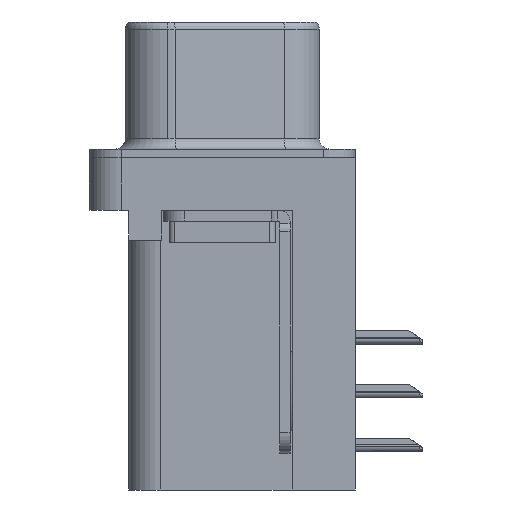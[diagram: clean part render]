
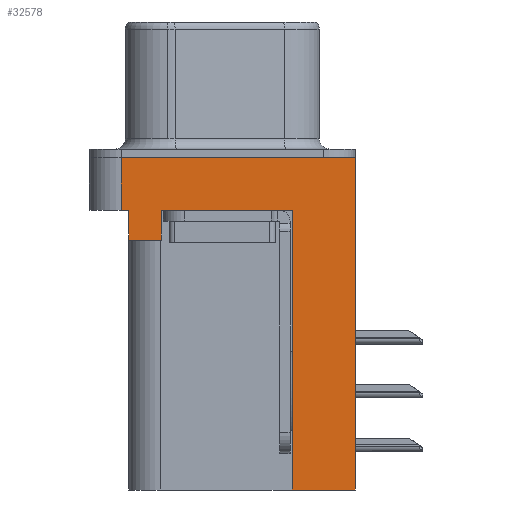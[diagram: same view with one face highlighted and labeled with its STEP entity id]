
A CAD part, left-side view. The second image highlights one B-rep face of the part: STEP entity #32578.
In plain terms, the highlighted planar face has unit normal (-1, 0, 0).
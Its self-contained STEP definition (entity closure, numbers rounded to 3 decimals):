
#447 = VERTEX_POINT ( 'NONE', #12961 ) ;
#768 = EDGE_CURVE ( 'NONE', #20074, #5395, #31731, .T. ) ;
#1675 = LINE ( 'NONE', #16676, #16002 ) ;
#2253 = ORIENTED_EDGE ( 'NONE', *, *, #27687, .T. ) ;
#2618 = ORIENTED_EDGE ( 'NONE', *, *, #26291, .F. ) ;
#2777 = DIRECTION ( 'NONE',  ( 0., 0., 1. ) ) ;
#2835 = CARTESIAN_POINT ( 'NONE',  ( -2.91, -6.275, -2.5 ) ) ;
#2850 = AXIS2_PLACEMENT_3D ( 'NONE', #2835, #25603, #8645 ) ;
#3186 = VECTOR ( 'NONE', #23266, 1000. ) ;
#3810 = LINE ( 'NONE', #24291, #19846 ) ;
#3878 = EDGE_CURVE ( 'NONE', #5395, #35663, #27976, .T. ) ;
#3960 = CARTESIAN_POINT ( 'NONE',  ( -2.91, -6.275, -2.5 ) ) ;
#4113 = LINE ( 'NONE', #3960, #33430 ) ;
#4437 = CARTESIAN_POINT ( 'NONE',  ( -2.91, -6.275, 0. ) ) ;
#5290 = DIRECTION ( 'NONE',  ( 0., 1., 0. ) ) ;
#5320 = EDGE_CURVE ( 'NONE', #447, #14655, #1675, .T. ) ;
#5395 = VERTEX_POINT ( 'NONE', #36560 ) ;
#5920 = VECTOR ( 'NONE', #34049, 1000. ) ;
#6061 = ORIENTED_EDGE ( 'NONE', *, *, #768, .F. ) ;
#6832 = LINE ( 'NONE', #25537, #5920 ) ;
#7365 = DIRECTION ( 'NONE',  ( 0., -1., 0. ) ) ;
#7595 = EDGE_CURVE ( 'NONE', #32643, #447, #21577, .T. ) ;
#7699 = LINE ( 'NONE', #20429, #3186 ) ;
#8645 = DIRECTION ( 'NONE',  ( 0., 0., 1. ) ) ;
#9405 = CARTESIAN_POINT ( 'NONE',  ( -2.91, 2.895, -3.9 ) ) ;
#10199 = DIRECTION ( 'NONE',  ( 0., -1., 0. ) ) ;
#10354 = CARTESIAN_POINT ( 'NONE',  ( -2.91, 4.425, -2.5 ) ) ;
#11674 = FACE_OUTER_BOUND ( 'NONE', #19146, .T. ) ;
#12716 = CARTESIAN_POINT ( 'NONE',  ( -2.91, -6.275, 0. ) ) ;
#12940 = VECTOR ( 'NONE', #7365, 1000. ) ;
#12961 = CARTESIAN_POINT ( 'NONE',  ( -2.91, -3.295, -15.7 ) ) ;
#13712 = DIRECTION ( 'NONE',  ( 0., 0., 1. ) ) ;
#13797 = VERTEX_POINT ( 'NONE', #10354 ) ;
#14472 = VERTEX_POINT ( 'NONE', #16010 ) ;
#14655 = VERTEX_POINT ( 'NONE', #36496 ) ;
#14767 = ORIENTED_EDGE ( 'NONE', *, *, #32955, .F. ) ;
#15121 = CARTESIAN_POINT ( 'NONE',  ( -2.91, 4.425, -3.9 ) ) ;
#16002 = VECTOR ( 'NONE', #13712, 1000. ) ;
#16010 = CARTESIAN_POINT ( 'NONE',  ( -2.91, 4.425, -3.9 ) ) ;
#16676 = CARTESIAN_POINT ( 'NONE',  ( -2.91, -3.295, -15.7 ) ) ;
#17444 = CARTESIAN_POINT ( 'NONE',  ( -2.91, -6.275, -15.7 ) ) ;
#19146 = EDGE_LOOP ( 'NONE', ( #26880, #6061, #21580, #2618, #14767, #2253, #30827, #32696, #29539, #23079 ) ) ;
#19846 = VECTOR ( 'NONE', #10199, 1000. ) ;
#20074 = VERTEX_POINT ( 'NONE', #29433 ) ;
#20429 = CARTESIAN_POINT ( 'NONE',  ( -2.91, -6.275, -2.5 ) ) ;
#20759 = DIRECTION ( 'NONE',  ( 0., 1., 0. ) ) ;
#21577 = LINE ( 'NONE', #28024, #29124 ) ;
#21580 = ORIENTED_EDGE ( 'NONE', *, *, #32000, .T. ) ;
#21582 = EDGE_CURVE ( 'NONE', #32643, #35663, #4113, .T. ) ;
#21803 = VECTOR ( 'NONE', #20759, 1000. ) ;
#22111 = CARTESIAN_POINT ( 'NONE',  ( -2.91, 2.895, -2.5 ) ) ;
#22682 = CARTESIAN_POINT ( 'NONE',  ( -2.91, 4.775, -2.5 ) ) ;
#22728 = PLANE ( 'NONE',  #2850 ) ;
#23079 = ORIENTED_EDGE ( 'NONE', *, *, #21582, .T. ) ;
#23266 = DIRECTION ( 'NONE',  ( 0., -1., 0. ) ) ;
#23990 = DIRECTION ( 'NONE',  ( 0., 0., 1. ) ) ;
#24088 = EDGE_CURVE ( 'NONE', #26711, #14655, #3810, .T. ) ;
#24199 = VECTOR ( 'NONE', #2777, 1000. ) ;
#24291 = CARTESIAN_POINT ( 'NONE',  ( -2.91, -6.275, -2.5 ) ) ;
#25293 = VERTEX_POINT ( 'NONE', #9405 ) ;
#25537 = CARTESIAN_POINT ( 'NONE',  ( -2.91, 4.425, -3.9 ) ) ;
#25603 = DIRECTION ( 'NONE',  ( -1., 0., 0. ) ) ;
#26291 = EDGE_CURVE ( 'NONE', #14472, #13797, #6832, .T. ) ;
#26711 = VERTEX_POINT ( 'NONE', #22111 ) ;
#26880 = ORIENTED_EDGE ( 'NONE', *, *, #3878, .F. ) ;
#27687 = EDGE_CURVE ( 'NONE', #25293, #26711, #34681, .T. ) ;
#27976 = LINE ( 'NONE', #4437, #12940 ) ;
#28024 = CARTESIAN_POINT ( 'NONE',  ( -2.91, -3.295, -15.7 ) ) ;
#29113 = CARTESIAN_POINT ( 'NONE',  ( -2.91, 2.895, -3.9 ) ) ;
#29124 = VECTOR ( 'NONE', #5290, 1000. ) ;
#29344 = LINE ( 'NONE', #15121, #21803 ) ;
#29433 = CARTESIAN_POINT ( 'NONE',  ( -2.91, 4.775, -2.5 ) ) ;
#29539 = ORIENTED_EDGE ( 'NONE', *, *, #7595, .F. ) ;
#30827 = ORIENTED_EDGE ( 'NONE', *, *, #24088, .T. ) ;
#31731 = LINE ( 'NONE', #22682, #24199 ) ;
#31958 = DIRECTION ( 'NONE',  ( 0., 0., 1. ) ) ;
#32000 = EDGE_CURVE ( 'NONE', #20074, #13797, #7699, .T. ) ;
#32578 = ADVANCED_FACE ( 'NONE', ( #11674 ), #22728, .T. ) ;
#32643 = VERTEX_POINT ( 'NONE', #17444 ) ;
#32696 = ORIENTED_EDGE ( 'NONE', *, *, #5320, .F. ) ;
#32955 = EDGE_CURVE ( 'NONE', #25293, #14472, #29344, .T. ) ;
#33430 = VECTOR ( 'NONE', #23990, 1000. ) ;
#33785 = VECTOR ( 'NONE', #31958, 1000. ) ;
#34049 = DIRECTION ( 'NONE',  ( 0., 0., 1. ) ) ;
#34681 = LINE ( 'NONE', #29113, #33785 ) ;
#35663 = VERTEX_POINT ( 'NONE', #12716 ) ;
#36496 = CARTESIAN_POINT ( 'NONE',  ( -2.91, -3.295, -2.5 ) ) ;
#36560 = CARTESIAN_POINT ( 'NONE',  ( -2.91, 4.775, 0. ) ) ;
